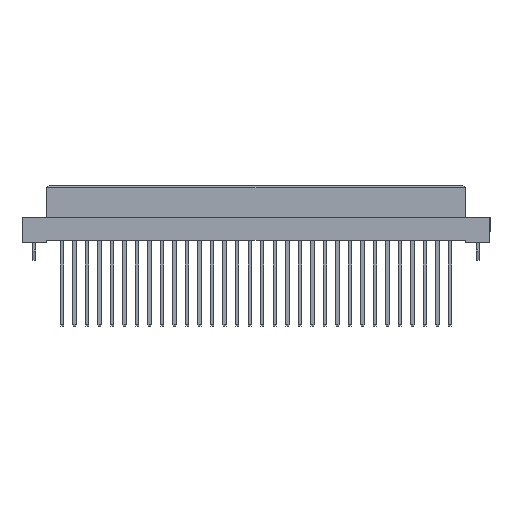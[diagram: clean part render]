
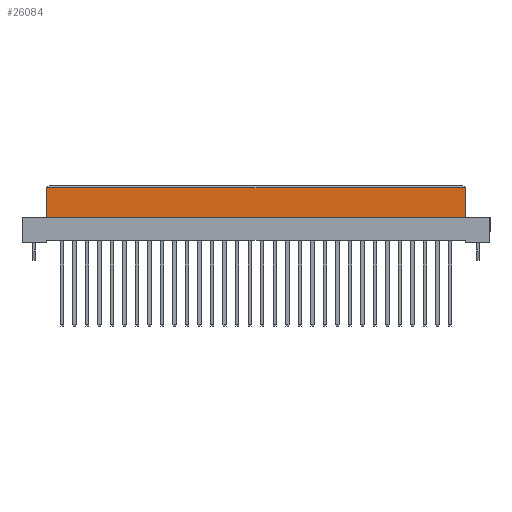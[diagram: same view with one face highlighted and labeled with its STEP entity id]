
A CAD part, top view. The second image highlights one B-rep face of the part: STEP entity #26084.
In plain terms, the highlighted planar face has unit normal (0, 0, 1).
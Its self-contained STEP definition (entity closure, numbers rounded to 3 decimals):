
#2593 = LINE ( 'NONE', #12245, #34490 ) ;
#3934 = EDGE_LOOP ( 'NONE', ( #5243, #36456, #33610, #5942 ) ) ;
#5243 = ORIENTED_EDGE ( 'NONE', *, *, #40735, .T. ) ;
#5432 = CARTESIAN_POINT ( 'NONE',  ( 42.5, -6.4, 4.25 ) ) ;
#5942 = ORIENTED_EDGE ( 'NONE', *, *, #12748, .T. ) ;
#7373 = EDGE_CURVE ( 'NONE', #26676, #21022, #2593, .T. ) ;
#7620 = CARTESIAN_POINT ( 'NONE',  ( 42.5, -6.4, 4.25 ) ) ;
#10409 = VERTEX_POINT ( 'NONE', #22071 ) ;
#11584 = DIRECTION ( 'NONE',  ( 1., 0., 0. ) ) ;
#11620 = VECTOR ( 'NONE', #11584, 1000. ) ;
#12245 = CARTESIAN_POINT ( 'NONE',  ( -42.5, -0.5, 4.25 ) ) ;
#12748 = EDGE_CURVE ( 'NONE', #10409, #19911, #33870, .T. ) ;
#14116 = CARTESIAN_POINT ( 'NONE',  ( -42.5, -6.4, 4.25 ) ) ;
#16646 = FACE_OUTER_BOUND ( 'NONE', #3934, .T. ) ;
#17618 = DIRECTION ( 'NONE',  ( 0., 1., 0. ) ) ;
#17703 = LINE ( 'NONE', #14116, #20835 ) ;
#18555 = CARTESIAN_POINT ( 'NONE',  ( 42.5, -6.4, 4.25 ) ) ;
#19911 = VERTEX_POINT ( 'NONE', #18555 ) ;
#20835 = VECTOR ( 'NONE', #29896, 1000. ) ;
#21022 = VERTEX_POINT ( 'NONE', #39003 ) ;
#21654 = AXIS2_PLACEMENT_3D ( 'NONE', #7620, #33036, #35989 ) ;
#21906 = DIRECTION ( 'NONE',  ( -1., 0., 0. ) ) ;
#22071 = CARTESIAN_POINT ( 'NONE',  ( -42.5, -6.4, 4.25 ) ) ;
#23181 = PLANE ( 'NONE',  #21654 ) ;
#23258 = EDGE_CURVE ( 'NONE', #10409, #21022, #17703, .T. ) ;
#26084 = ADVANCED_FACE ( 'NONE', ( #16646 ), #23181, .T. ) ;
#26676 = VERTEX_POINT ( 'NONE', #38579 ) ;
#27549 = CARTESIAN_POINT ( 'NONE',  ( 42.5, -6.4, 4.25 ) ) ;
#29896 = DIRECTION ( 'NONE',  ( 0., 1., 0. ) ) ;
#30659 = LINE ( 'NONE', #5432, #31930 ) ;
#31930 = VECTOR ( 'NONE', #17618, 1000. ) ;
#33036 = DIRECTION ( 'NONE',  ( 0., 0., 1. ) ) ;
#33610 = ORIENTED_EDGE ( 'NONE', *, *, #23258, .F. ) ;
#33870 = LINE ( 'NONE', #27549, #11620 ) ;
#34490 = VECTOR ( 'NONE', #21906, 1000. ) ;
#35989 = DIRECTION ( 'NONE',  ( 1., 0., 0. ) ) ;
#36456 = ORIENTED_EDGE ( 'NONE', *, *, #7373, .T. ) ;
#38579 = CARTESIAN_POINT ( 'NONE',  ( 42.5, -0.5, 4.25 ) ) ;
#39003 = CARTESIAN_POINT ( 'NONE',  ( -42.5, -0.5, 4.25 ) ) ;
#40735 = EDGE_CURVE ( 'NONE', #19911, #26676, #30659, .T. ) ;
